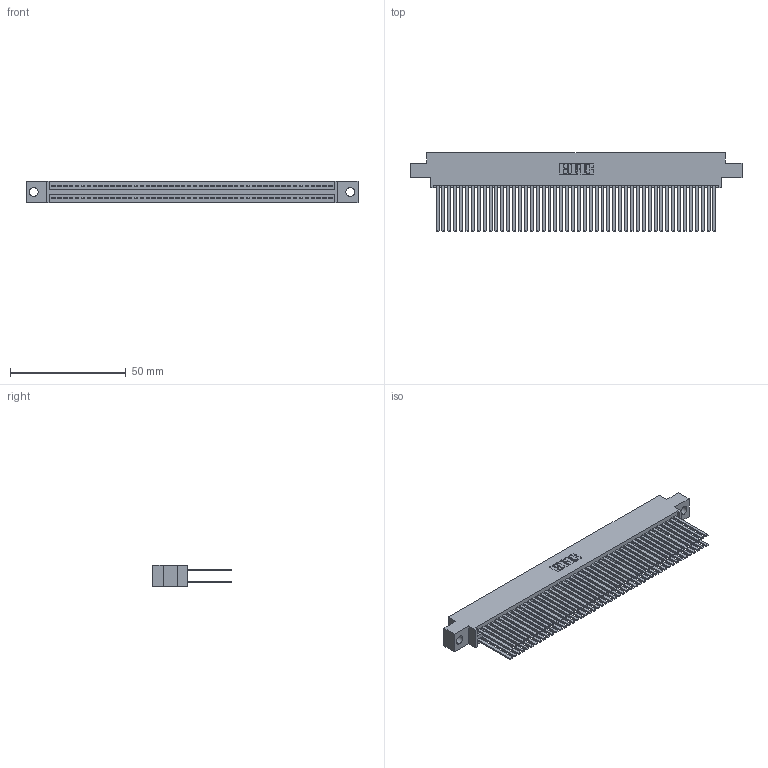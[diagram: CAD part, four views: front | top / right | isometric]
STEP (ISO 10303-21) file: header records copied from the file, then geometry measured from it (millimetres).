
FILE_DESCRIPTION (( 'STEP AP203' ), '1' );
FILE_NAME ('395-096-544-804.STEP', '2018-11-29T16:28:43', ( '' ), ( '' ), 'SwSTEP 2.0', 'SolidWorks 2016', '' );
FILE_SCHEMA (( 'CONFIG_CONTROL_DESIGN' ));
Length unit declared in the file: inch
Products named in the file (3): 345-292-001_345-293-144; 345 Part_0.170 Offset - 0.156 Dia-TH; 395-096-544-804
Assembly tree (97 placements, depth 2):
  395-096-544-804
    345 Part_0.170 Offset - 0.156 Dia-TH
    345-292-001_345-293-144  x96
Bounding box: 143.13 x 33.96 x 9.4 mm (x, y, z)
Volume: 15103.9 mm3; surface area: 26345.2 mm2
Topology: 97 solids, 97 shells, 4354 faces, 12929 edges, 8490 vertices
Faces by surface type: plane 2868, cylinder 1486
Entity records: 36805 total; most frequent: CARTESIAN_POINT 6164, ORIENTED_EDGE 6098, DIRECTION 5425, EDGE_CURVE 3049, LINE 2729, VECTOR 2729, VERTEX_POINT 2030, AXIS2_PLACEMENT_3D 1348
